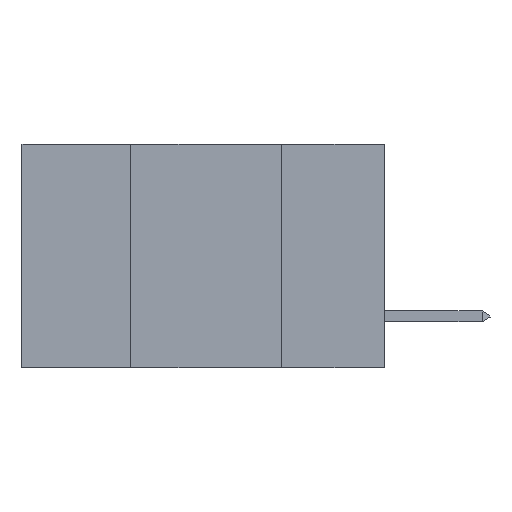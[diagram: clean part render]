
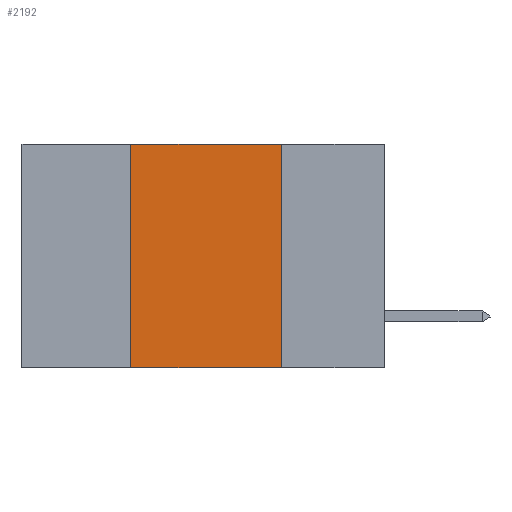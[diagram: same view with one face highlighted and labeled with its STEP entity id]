
A CAD part, left-side view. The second image highlights one B-rep face of the part: STEP entity #2192.
In plain terms, the highlighted planar face has unit normal (-1, 0, 0).
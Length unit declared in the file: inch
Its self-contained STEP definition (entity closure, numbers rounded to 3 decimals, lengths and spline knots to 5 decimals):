
#15 = DIRECTION ( 'NONE',  ( 1., 0., 0. ) ) ;
#1192 = EDGE_CURVE ( 'NONE', #31637, #32779, #30932, .T. ) ;
#2192 = ADVANCED_FACE ( 'NONE', ( #16850 ), #27625, .F. ) ;
#4406 = EDGE_CURVE ( 'NONE', #28782, #31637, #21473, .T. ) ;
#5113 = DIRECTION ( 'NONE',  ( 0., 0., -1. ) ) ;
#6713 = CARTESIAN_POINT ( 'NONE',  ( 0., 0.6, 0. ) ) ;
#7112 = EDGE_CURVE ( 'NONE', #28676, #28782, #32489, .T. ) ;
#10443 = ORIENTED_EDGE ( 'NONE', *, *, #4406, .F. ) ;
#12512 = CARTESIAN_POINT ( 'NONE',  ( 0., 0.42, 0. ) ) ;
#13194 = CARTESIAN_POINT ( 'NONE',  ( 0., 0.17, 0. ) ) ;
#15609 = CARTESIAN_POINT ( 'NONE',  ( 0., 0.6, -0.37 ) ) ;
#16850 = FACE_OUTER_BOUND ( 'NONE', #29616, .T. ) ;
#18403 = CARTESIAN_POINT ( 'NONE',  ( 0., 0.17, 0. ) ) ;
#20571 = CARTESIAN_POINT ( 'NONE',  ( 0., 0.42, -0.37 ) ) ;
#20765 = DIRECTION ( 'NONE',  ( 0., 0., 1. ) ) ;
#21368 = DIRECTION ( 'NONE',  ( 0., -1., 0. ) ) ;
#21473 = LINE ( 'NONE', #21518, #26364 ) ;
#21518 = CARTESIAN_POINT ( 'NONE',  ( 0., 0.6, 0. ) ) ;
#22886 = DIRECTION ( 'NONE',  ( 0., -1., 0. ) ) ;
#24751 = DIRECTION ( 'NONE',  ( 0., 0., -1. ) ) ;
#24857 = VECTOR ( 'NONE', #22886, 39.37008 ) ;
#24917 = ORIENTED_EDGE ( 'NONE', *, *, #38013, .T. ) ;
#25892 = AXIS2_PLACEMENT_3D ( 'NONE', #6713, #15, #24751 ) ;
#26364 = VECTOR ( 'NONE', #21368, 39.37008 ) ;
#27625 = PLANE ( 'NONE',  #25892 ) ;
#28191 = CARTESIAN_POINT ( 'NONE',  ( 0., 0.42, 0. ) ) ;
#28676 = VERTEX_POINT ( 'NONE', #20571 ) ;
#28782 = VERTEX_POINT ( 'NONE', #12512 ) ;
#29616 = EDGE_LOOP ( 'NONE', ( #34900, #10443, #34199, #24917 ) ) ;
#30932 = LINE ( 'NONE', #18403, #43385 ) ;
#31637 = VERTEX_POINT ( 'NONE', #13194 ) ;
#32489 = LINE ( 'NONE', #28191, #43279 ) ;
#32779 = VERTEX_POINT ( 'NONE', #43267 ) ;
#34199 = ORIENTED_EDGE ( 'NONE', *, *, #7112, .F. ) ;
#34900 = ORIENTED_EDGE ( 'NONE', *, *, #1192, .F. ) ;
#38013 = EDGE_CURVE ( 'NONE', #28676, #32779, #38318, .T. ) ;
#38318 = LINE ( 'NONE', #15609, #24857 ) ;
#43267 = CARTESIAN_POINT ( 'NONE',  ( 0., 0.17, -0.37 ) ) ;
#43279 = VECTOR ( 'NONE', #20765, 39.37008 ) ;
#43385 = VECTOR ( 'NONE', #5113, 39.37008 ) ;
